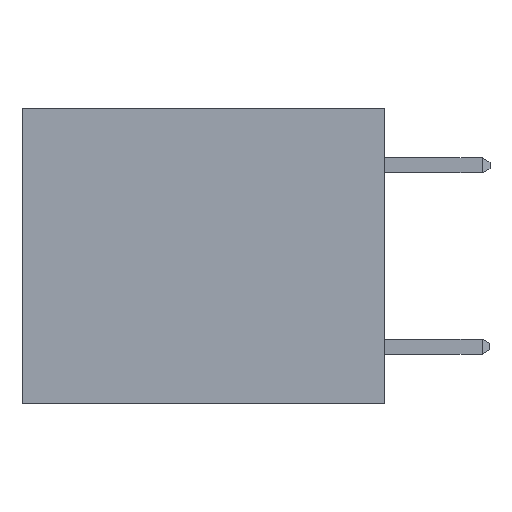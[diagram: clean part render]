
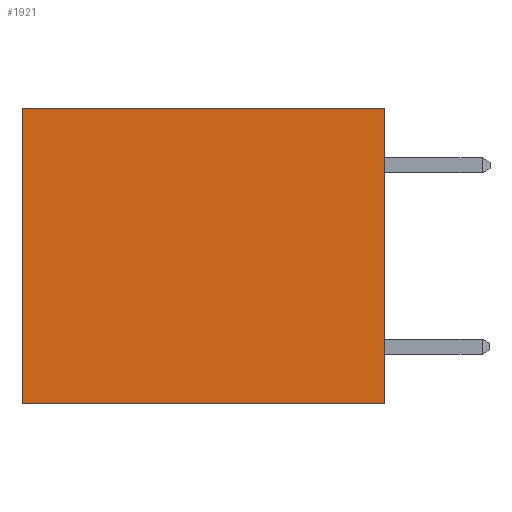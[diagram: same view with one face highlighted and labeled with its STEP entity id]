
A CAD part, left-side view. The second image highlights one B-rep face of the part: STEP entity #1921.
In plain terms, the highlighted planar face has unit normal (-1, 0, 0).
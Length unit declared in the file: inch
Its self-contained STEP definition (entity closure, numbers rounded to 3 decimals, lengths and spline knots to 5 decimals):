
#320 = ORIENTED_EDGE ( 'NONE', *, *, #7610, .F. ) ;
#585 = CARTESIAN_POINT ( 'NONE',  ( 0.3165, 0., -0.49 ) ) ;
#607 = DIRECTION ( 'NONE',  ( 0., 0., -1. ) ) ;
#737 = CARTESIAN_POINT ( 'NONE',  ( 0.3165, 0.6, -0.49 ) ) ;
#787 = LINE ( 'NONE', #2195, #4897 ) ;
#977 = AXIS2_PLACEMENT_3D ( 'NONE', #4501, #2824, #607 ) ;
#1103 = LINE ( 'NONE', #585, #1379 ) ;
#1321 = LINE ( 'NONE', #7438, #6587 ) ;
#1379 = VECTOR ( 'NONE', #3019, 39.37008 ) ;
#1921 = ADVANCED_FACE ( 'NONE', ( #2586 ), #6858, .F. ) ;
#2195 = CARTESIAN_POINT ( 'NONE',  ( 0.3165, 0.6, -0.49 ) ) ;
#2241 = VECTOR ( 'NONE', #3923, 39.37008 ) ;
#2461 = VERTEX_POINT ( 'NONE', #2554 ) ;
#2554 = CARTESIAN_POINT ( 'NONE',  ( 0.3165, 0., 0. ) ) ;
#2586 = FACE_OUTER_BOUND ( 'NONE', #4094, .T. ) ;
#2736 = ORIENTED_EDGE ( 'NONE', *, *, #5275, .T. ) ;
#2824 = DIRECTION ( 'NONE',  ( 1., 0., 0. ) ) ;
#3019 = DIRECTION ( 'NONE',  ( 0., 1., 0. ) ) ;
#3468 = CARTESIAN_POINT ( 'NONE',  ( 0.3165, 0.6, 0. ) ) ;
#3553 = ORIENTED_EDGE ( 'NONE', *, *, #5655, .F. ) ;
#3923 = DIRECTION ( 'NONE',  ( 0., 0., -1. ) ) ;
#4094 = EDGE_LOOP ( 'NONE', ( #2736, #320, #3553, #4348 ) ) ;
#4348 = ORIENTED_EDGE ( 'NONE', *, *, #5570, .T. ) ;
#4501 = CARTESIAN_POINT ( 'NONE',  ( 0.3165, 0., -0.49 ) ) ;
#4897 = VECTOR ( 'NONE', #7016, 39.37008 ) ;
#5028 = VERTEX_POINT ( 'NONE', #737 ) ;
#5275 = EDGE_CURVE ( 'NONE', #6512, #5028, #787, .T. ) ;
#5457 = LINE ( 'NONE', #6904, #2241 ) ;
#5570 = EDGE_CURVE ( 'NONE', #2461, #6512, #1321, .T. ) ;
#5655 = EDGE_CURVE ( 'NONE', #2461, #6890, #5457, .T. ) ;
#5679 = DIRECTION ( 'NONE',  ( 0., 1., 0. ) ) ;
#6512 = VERTEX_POINT ( 'NONE', #3468 ) ;
#6587 = VECTOR ( 'NONE', #5679, 39.37008 ) ;
#6858 = PLANE ( 'NONE',  #977 ) ;
#6890 = VERTEX_POINT ( 'NONE', #7559 ) ;
#6904 = CARTESIAN_POINT ( 'NONE',  ( 0.3165, 0., -0.49 ) ) ;
#7016 = DIRECTION ( 'NONE',  ( 0., 0., -1. ) ) ;
#7438 = CARTESIAN_POINT ( 'NONE',  ( 0.3165, 0., 0. ) ) ;
#7559 = CARTESIAN_POINT ( 'NONE',  ( 0.3165, 0., -0.49 ) ) ;
#7610 = EDGE_CURVE ( 'NONE', #6890, #5028, #1103, .T. ) ;
